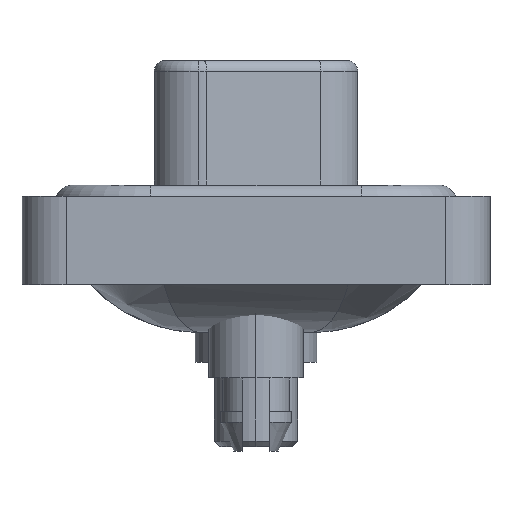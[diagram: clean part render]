
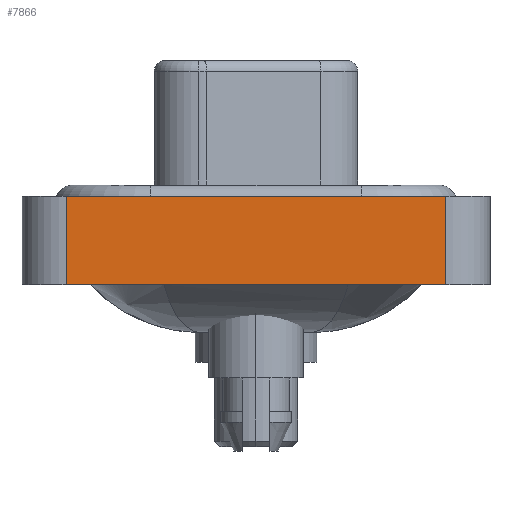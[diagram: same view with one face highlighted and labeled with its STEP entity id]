
A CAD part, left-side view. The second image highlights one B-rep face of the part: STEP entity #7866.
In plain terms, the highlighted planar face has unit normal (-1, 0, 0).
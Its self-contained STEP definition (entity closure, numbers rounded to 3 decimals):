
#1218 = CARTESIAN_POINT ( 'NONE',  ( -7.3, -8.55, -3.6 ) ) ;
#1671 = VERTEX_POINT ( 'NONE', #9023 ) ;
#1909 = CARTESIAN_POINT ( 'NONE',  ( -7.3, 8.55, -3.6 ) ) ;
#2486 = LINE ( 'NONE', #8686, #5073 ) ;
#2523 = EDGE_CURVE ( 'NONE', #8961, #6477, #8795, .T. ) ;
#2753 = ORIENTED_EDGE ( 'NONE', *, *, #4337, .F. ) ;
#3253 = LINE ( 'NONE', #1909, #5841 ) ;
#3433 = EDGE_CURVE ( 'NONE', #6477, #14632, #19740, .T. ) ;
#4276 = DIRECTION ( 'NONE',  ( 0., 0., 1. ) ) ;
#4337 = EDGE_CURVE ( 'NONE', #8961, #1671, #3253, .T. ) ;
#5073 = VECTOR ( 'NONE', #13129, 1000. ) ;
#5841 = VECTOR ( 'NONE', #17399, 1000. ) ;
#6113 = EDGE_CURVE ( 'NONE', #1671, #14632, #2486, .T. ) ;
#6141 = ORIENTED_EDGE ( 'NONE', *, *, #6113, .F. ) ;
#6477 = VERTEX_POINT ( 'NONE', #16351 ) ;
#7141 = CARTESIAN_POINT ( 'NONE',  ( -7.3, -8.55, 0.4 ) ) ;
#7177 = CARTESIAN_POINT ( 'NONE',  ( -7.3, -8.55, -3.6 ) ) ;
#7405 = DIRECTION ( 'NONE',  ( 0., 0., 1. ) ) ;
#7866 = ADVANCED_FACE ( 'NONE', ( #15182 ), #15080, .T. ) ;
#8562 = CARTESIAN_POINT ( 'NONE',  ( -7.3, 8.55, -3.6 ) ) ;
#8686 = CARTESIAN_POINT ( 'NONE',  ( -7.3, -8.55, 0.4 ) ) ;
#8795 = LINE ( 'NONE', #7177, #9461 ) ;
#8961 = VERTEX_POINT ( 'NONE', #8562 ) ;
#9023 = CARTESIAN_POINT ( 'NONE',  ( -7.3, 8.55, 0.4 ) ) ;
#9461 = VECTOR ( 'NONE', #16664, 1000. ) ;
#9827 = EDGE_LOOP ( 'NONE', ( #10277, #6141, #2753, #19407 ) ) ;
#10277 = ORIENTED_EDGE ( 'NONE', *, *, #3433, .T. ) ;
#10627 = CARTESIAN_POINT ( 'NONE',  ( -7.3, -8.55, -3.6 ) ) ;
#12922 = AXIS2_PLACEMENT_3D ( 'NONE', #1218, #13680, #7405 ) ;
#13129 = DIRECTION ( 'NONE',  ( 0., -1., 0. ) ) ;
#13680 = DIRECTION ( 'NONE',  ( -1., 0., 0. ) ) ;
#14632 = VERTEX_POINT ( 'NONE', #7141 ) ;
#15080 = PLANE ( 'NONE',  #12922 ) ;
#15182 = FACE_OUTER_BOUND ( 'NONE', #9827, .T. ) ;
#16351 = CARTESIAN_POINT ( 'NONE',  ( -7.3, -8.55, -3.6 ) ) ;
#16664 = DIRECTION ( 'NONE',  ( 0., -1., 0. ) ) ;
#17231 = VECTOR ( 'NONE', #4276, 1000. ) ;
#17399 = DIRECTION ( 'NONE',  ( 0., 0., 1. ) ) ;
#19407 = ORIENTED_EDGE ( 'NONE', *, *, #2523, .T. ) ;
#19740 = LINE ( 'NONE', #10627, #17231 ) ;
